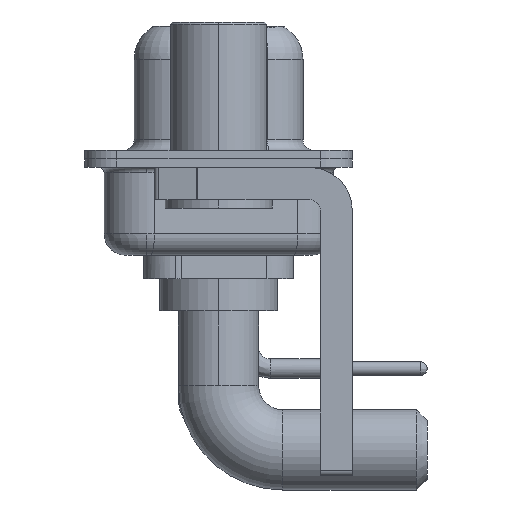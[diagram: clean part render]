
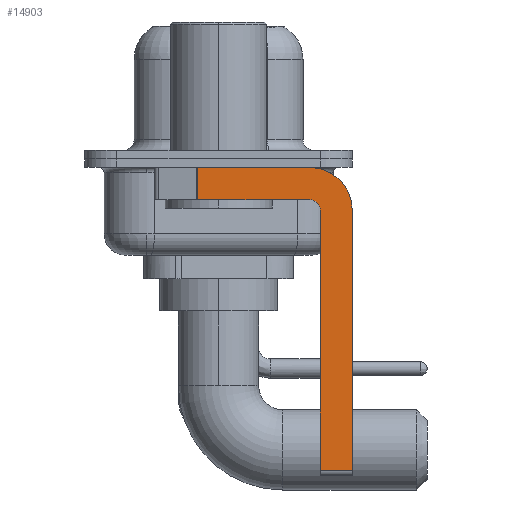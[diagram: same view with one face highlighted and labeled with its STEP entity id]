
A CAD part, left-side view. The second image highlights one B-rep face of the part: STEP entity #14903.
In plain terms, the highlighted planar face has unit normal (-1, 0, 0).
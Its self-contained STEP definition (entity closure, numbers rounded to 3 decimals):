
#703 = EDGE_LOOP ( 'NONE', ( #2973, #12882, #14984, #13126, #11957, #6969, #5052, #12483 ) ) ;
#773 = VERTEX_POINT ( 'NONE', #6326 ) ;
#983 = VECTOR ( 'NONE', #5213, 1000. ) ;
#984 = VECTOR ( 'NONE', #15874, 1000. ) ;
#1033 = EDGE_CURVE ( 'NONE', #8335, #16180, #9998, .T. ) ;
#1132 = CARTESIAN_POINT ( 'NONE',  ( -2.9, -6.25, -14.55 ) ) ;
#1158 = VERTEX_POINT ( 'NONE', #6099 ) ;
#2973 = ORIENTED_EDGE ( 'NONE', *, *, #10903, .F. ) ;
#3500 = VERTEX_POINT ( 'NONE', #18002 ) ;
#3700 = CARTESIAN_POINT ( 'NONE',  ( -2.9, -4.25, -14.55 ) ) ;
#3997 = EDGE_CURVE ( 'NONE', #1158, #773, #19562, .T. ) ;
#4008 = VECTOR ( 'NONE', #8809, 1000. ) ;
#4138 = VECTOR ( 'NONE', #14931, 1000. ) ;
#4753 = CARTESIAN_POINT ( 'NONE',  ( -2.9, -4.25, -0.4 ) ) ;
#5052 = ORIENTED_EDGE ( 'NONE', *, *, #13472, .F. ) ;
#5213 = DIRECTION ( 'NONE',  ( 0., -1., 0. ) ) ;
#5933 = LINE ( 'NONE', #9228, #10677 ) ;
#6037 = LINE ( 'NONE', #7344, #4138 ) ;
#6038 = EDGE_CURVE ( 'NONE', #12656, #3500, #6676, .T. ) ;
#6099 = CARTESIAN_POINT ( 'NONE',  ( -2.9, -4.75, -14.55 ) ) ;
#6306 = CARTESIAN_POINT ( 'NONE',  ( -2.9, -4.25, -2.4 ) ) ;
#6326 = CARTESIAN_POINT ( 'NONE',  ( -2.9, -4.75, -2.4 ) ) ;
#6676 = CIRCLE ( 'NONE', #15612, 2. ) ;
#6969 = ORIENTED_EDGE ( 'NONE', *, *, #14630, .T. ) ;
#7011 = CARTESIAN_POINT ( 'NONE',  ( -2.9, -4.25, -1.9 ) ) ;
#7344 = CARTESIAN_POINT ( 'NONE',  ( -2.9, 3., -0.4 ) ) ;
#7530 = EDGE_CURVE ( 'NONE', #773, #8335, #15297, .T. ) ;
#8335 = VERTEX_POINT ( 'NONE', #11207 ) ;
#8809 = DIRECTION ( 'NONE',  ( 0., 1., 0. ) ) ;
#8819 = CARTESIAN_POINT ( 'NONE',  ( -2.9, 0.978, -0.4 ) ) ;
#9228 = CARTESIAN_POINT ( 'NONE',  ( -2.9, 0.978, -1.9 ) ) ;
#9563 = CARTESIAN_POINT ( 'NONE',  ( -2.9, -4.25, -2.4 ) ) ;
#9754 = CARTESIAN_POINT ( 'NONE',  ( -2.9, -6.25, -2.4 ) ) ;
#9998 = LINE ( 'NONE', #7011, #4008 ) ;
#10550 = CARTESIAN_POINT ( 'NONE',  ( -2.9, -4.75, -14.8 ) ) ;
#10677 = VECTOR ( 'NONE', #16738, 1000. ) ;
#10707 = VERTEX_POINT ( 'NONE', #1132 ) ;
#10892 = DIRECTION ( 'NONE',  ( 1., 0., 0. ) ) ;
#10903 = EDGE_CURVE ( 'NONE', #18191, #12656, #6037, .T. ) ;
#11207 = CARTESIAN_POINT ( 'NONE',  ( -2.9, -4.25, -1.9 ) ) ;
#11253 = LINE ( 'NONE', #9754, #984 ) ;
#11957 = ORIENTED_EDGE ( 'NONE', *, *, #3997, .F. ) ;
#12483 = ORIENTED_EDGE ( 'NONE', *, *, #6038, .F. ) ;
#12559 = DIRECTION ( 'NONE',  ( 1., 0., 0. ) ) ;
#12656 = VERTEX_POINT ( 'NONE', #4753 ) ;
#12735 = AXIS2_PLACEMENT_3D ( 'NONE', #9563, #14455, #18685 ) ;
#12882 = ORIENTED_EDGE ( 'NONE', *, *, #17896, .T. ) ;
#13126 = ORIENTED_EDGE ( 'NONE', *, *, #7530, .F. ) ;
#13472 = EDGE_CURVE ( 'NONE', #3500, #10707, #11253, .T. ) ;
#13704 = CARTESIAN_POINT ( 'NONE',  ( -2.9, 0.978, -1.9 ) ) ;
#13897 = DIRECTION ( 'NONE',  ( 0., 0., -1. ) ) ;
#14403 = LINE ( 'NONE', #3700, #983 ) ;
#14450 = CARTESIAN_POINT ( 'NONE',  ( -2.9, -4.25, -2.4 ) ) ;
#14455 = DIRECTION ( 'NONE',  ( -1., 0., 0. ) ) ;
#14630 = EDGE_CURVE ( 'NONE', #1158, #10707, #14403, .T. ) ;
#14903 = ADVANCED_FACE ( 'NONE', ( #18714 ), #16806, .F. ) ;
#14931 = DIRECTION ( 'NONE',  ( 0., -1., 0. ) ) ;
#14984 = ORIENTED_EDGE ( 'NONE', *, *, #1033, .F. ) ;
#15297 = CIRCLE ( 'NONE', #12735, 0.5 ) ;
#15612 = AXIS2_PLACEMENT_3D ( 'NONE', #14450, #12559, #17272 ) ;
#15874 = DIRECTION ( 'NONE',  ( 0., 0., -1. ) ) ;
#15895 = VECTOR ( 'NONE', #16662, 1000. ) ;
#16180 = VERTEX_POINT ( 'NONE', #13704 ) ;
#16662 = DIRECTION ( 'NONE',  ( 0., 0., 1. ) ) ;
#16738 = DIRECTION ( 'NONE',  ( 0., 0., -1. ) ) ;
#16806 = PLANE ( 'NONE',  #19192 ) ;
#17272 = DIRECTION ( 'NONE',  ( 0., 0., -1. ) ) ;
#17896 = EDGE_CURVE ( 'NONE', #18191, #16180, #5933, .T. ) ;
#18002 = CARTESIAN_POINT ( 'NONE',  ( -2.9, -6.25, -2.4 ) ) ;
#18191 = VERTEX_POINT ( 'NONE', #8819 ) ;
#18685 = DIRECTION ( 'NONE',  ( 0., 0., 1. ) ) ;
#18714 = FACE_OUTER_BOUND ( 'NONE', #703, .T. ) ;
#19192 = AXIS2_PLACEMENT_3D ( 'NONE', #6306, #10892, #13897 ) ;
#19562 = LINE ( 'NONE', #10550, #15895 ) ;
